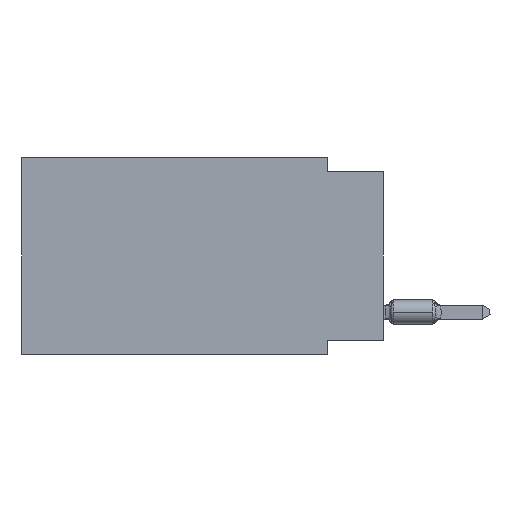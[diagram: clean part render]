
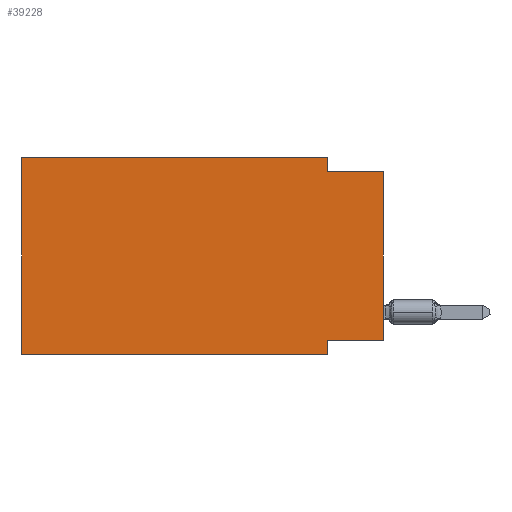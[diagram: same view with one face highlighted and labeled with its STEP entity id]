
A CAD part, left-side view. The second image highlights one B-rep face of the part: STEP entity #39228.
In plain terms, the highlighted planar face has unit normal (-1, 0, 0).
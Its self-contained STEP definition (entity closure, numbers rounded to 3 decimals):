
#160 = VERTEX_POINT ( 'NONE', #28824 ) ;
#761 = LINE ( 'NONE', #11258, #27602 ) ;
#1681 = CARTESIAN_POINT ( 'NONE',  ( 0., 0., 0. ) ) ;
#1999 = VERTEX_POINT ( 'NONE', #22640 ) ;
#3599 = CARTESIAN_POINT ( 'NONE',  ( 0., 16.383, 0. ) ) ;
#4616 = DIRECTION ( 'NONE',  ( 1., 0., 0. ) ) ;
#5635 = LINE ( 'NONE', #1681, #16174 ) ;
#7152 = VERTEX_POINT ( 'NONE', #52669 ) ;
#7348 = ORIENTED_EDGE ( 'NONE', *, *, #24824, .F. ) ;
#9523 = DIRECTION ( 'NONE',  ( 0., 0., -1. ) ) ;
#10437 = DIRECTION ( 'NONE',  ( 0., -1., 0. ) ) ;
#11258 = CARTESIAN_POINT ( 'NONE',  ( 0., 2.54, -8.89 ) ) ;
#11353 = ORIENTED_EDGE ( 'NONE', *, *, #36988, .T. ) ;
#12748 = ORIENTED_EDGE ( 'NONE', *, *, #14566, .F. ) ;
#13948 = CARTESIAN_POINT ( 'NONE',  ( 0., 0., -8.255 ) ) ;
#14052 = DIRECTION ( 'NONE',  ( 0., -1., 0. ) ) ;
#14440 = FACE_OUTER_BOUND ( 'NONE', #28228, .T. ) ;
#14566 = EDGE_CURVE ( 'NONE', #160, #19404, #33542, .T. ) ;
#14891 = AXIS2_PLACEMENT_3D ( 'NONE', #53462, #4616, #9523 ) ;
#16174 = VECTOR ( 'NONE', #21710, 1000. ) ;
#18873 = DIRECTION ( 'NONE',  ( 0., 1., 0. ) ) ;
#19404 = VERTEX_POINT ( 'NONE', #3599 ) ;
#21710 = DIRECTION ( 'NONE',  ( 0., 0., 1. ) ) ;
#22545 = VERTEX_POINT ( 'NONE', #24322 ) ;
#22640 = CARTESIAN_POINT ( 'NONE',  ( 0., 2.54, -8.89 ) ) ;
#24322 = CARTESIAN_POINT ( 'NONE',  ( 0., 2.54, 0. ) ) ;
#24824 = EDGE_CURVE ( 'NONE', #7152, #1999, #761, .T. ) ;
#27602 = VECTOR ( 'NONE', #50605, 1000. ) ;
#28228 = EDGE_LOOP ( 'NONE', ( #56174, #57456, #56679, #45421, #12748, #11353, #7348, #34256 ) ) ;
#28824 = CARTESIAN_POINT ( 'NONE',  ( 0., 16.383, -8.89 ) ) ;
#30193 = EDGE_CURVE ( 'NONE', #19404, #22545, #58951, .T. ) ;
#31661 = EDGE_CURVE ( 'NONE', #56866, #55958, #35371, .T. ) ;
#32713 = VECTOR ( 'NONE', #62275, 1000. ) ;
#33542 = LINE ( 'NONE', #57144, #56306 ) ;
#34256 = ORIENTED_EDGE ( 'NONE', *, *, #62115, .F. ) ;
#35371 = LINE ( 'NONE', #55331, #48095 ) ;
#36988 = EDGE_CURVE ( 'NONE', #160, #1999, #61950, .T. ) ;
#38265 = CARTESIAN_POINT ( 'NONE',  ( 0., 2.54, 0. ) ) ;
#39228 = ADVANCED_FACE ( 'NONE', ( #14440 ), #39380, .F. ) ;
#39380 = PLANE ( 'NONE',  #14891 ) ;
#41159 = EDGE_CURVE ( 'NONE', #57975, #55958, #5635, .T. ) ;
#42316 = CARTESIAN_POINT ( 'NONE',  ( 0., 16.383, -8.89 ) ) ;
#45336 = EDGE_CURVE ( 'NONE', #22545, #56866, #64091, .T. ) ;
#45421 = ORIENTED_EDGE ( 'NONE', *, *, #30193, .F. ) ;
#48095 = VECTOR ( 'NONE', #10437, 1000. ) ;
#48292 = DIRECTION ( 'NONE',  ( 0., 0., 1. ) ) ;
#49158 = VECTOR ( 'NONE', #14052, 1000. ) ;
#50605 = DIRECTION ( 'NONE',  ( 0., 0., -1. ) ) ;
#51123 = CARTESIAN_POINT ( 'NONE',  ( 0., 2.54, -0.635 ) ) ;
#51487 = VECTOR ( 'NONE', #53291, 1000. ) ;
#52669 = CARTESIAN_POINT ( 'NONE',  ( 0., 2.54, -8.255 ) ) ;
#53291 = DIRECTION ( 'NONE',  ( 0., 0., -1. ) ) ;
#53462 = CARTESIAN_POINT ( 'NONE',  ( 0., 16.383, 0. ) ) ;
#54139 = VECTOR ( 'NONE', #18873, 1000. ) ;
#55331 = CARTESIAN_POINT ( 'NONE',  ( 0., 0., -0.635 ) ) ;
#55958 = VERTEX_POINT ( 'NONE', #64146 ) ;
#56174 = ORIENTED_EDGE ( 'NONE', *, *, #41159, .T. ) ;
#56306 = VECTOR ( 'NONE', #48292, 1000. ) ;
#56679 = ORIENTED_EDGE ( 'NONE', *, *, #45336, .F. ) ;
#56866 = VERTEX_POINT ( 'NONE', #51123 ) ;
#57144 = CARTESIAN_POINT ( 'NONE',  ( 0., 16.383, 0. ) ) ;
#57456 = ORIENTED_EDGE ( 'NONE', *, *, #31661, .F. ) ;
#57975 = VERTEX_POINT ( 'NONE', #60823 ) ;
#58853 = LINE ( 'NONE', #13948, #54139 ) ;
#58951 = LINE ( 'NONE', #64497, #49158 ) ;
#60823 = CARTESIAN_POINT ( 'NONE',  ( 0., 0., -8.255 ) ) ;
#61950 = LINE ( 'NONE', #42316, #32713 ) ;
#62115 = EDGE_CURVE ( 'NONE', #57975, #7152, #58853, .T. ) ;
#62275 = DIRECTION ( 'NONE',  ( 0., -1., 0. ) ) ;
#64091 = LINE ( 'NONE', #38265, #51487 ) ;
#64146 = CARTESIAN_POINT ( 'NONE',  ( 0., 0., -0.635 ) ) ;
#64497 = CARTESIAN_POINT ( 'NONE',  ( 0., 16.383, 0. ) ) ;
